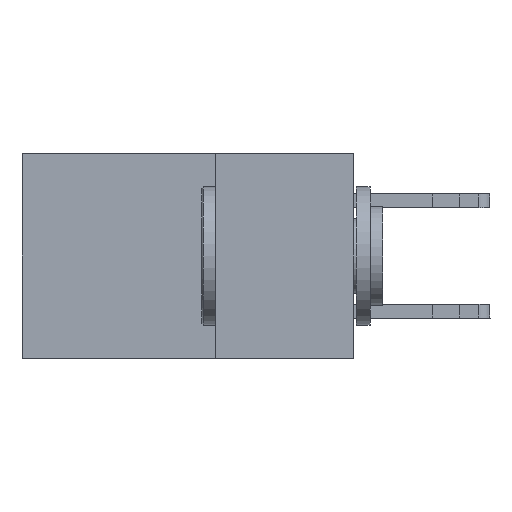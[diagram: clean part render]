
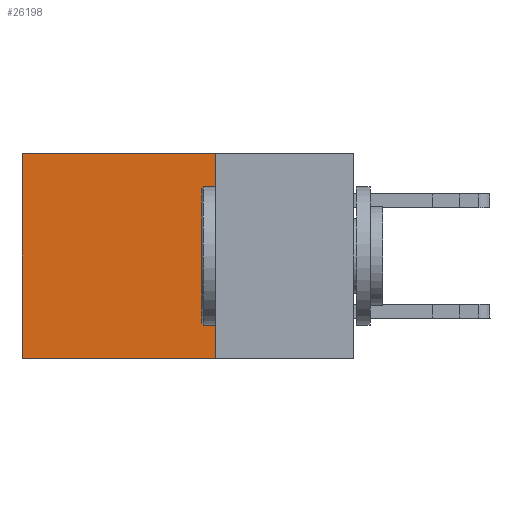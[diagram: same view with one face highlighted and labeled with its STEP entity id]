
A CAD part, left-side view. The second image highlights one B-rep face of the part: STEP entity #26198.
In plain terms, the highlighted planar face has unit normal (-1, 0, 0).
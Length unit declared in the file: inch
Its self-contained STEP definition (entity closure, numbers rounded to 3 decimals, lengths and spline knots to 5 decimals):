
#371 = CARTESIAN_POINT ( 'NONE',  ( 0.2875, 0.25, 0. ) ) ;
#1113 = LINE ( 'NONE', #1233, #7496 ) ;
#1233 = CARTESIAN_POINT ( 'NONE',  ( 0.2875, 0.6, 0. ) ) ;
#1409 = VERTEX_POINT ( 'NONE', #371 ) ;
#1474 = EDGE_CURVE ( 'NONE', #1409, #21731, #23817, .T. ) ;
#1758 = DIRECTION ( 'NONE',  ( 0., 1., 0. ) ) ;
#2656 = VERTEX_POINT ( 'NONE', #4469 ) ;
#2850 = DIRECTION ( 'NONE',  ( 0., 0., -1. ) ) ;
#3101 = LINE ( 'NONE', #16867, #10256 ) ;
#4096 = CARTESIAN_POINT ( 'NONE',  ( 0.2875, 0.25, -0.37 ) ) ;
#4252 = LINE ( 'NONE', #26974, #12473 ) ;
#4469 = CARTESIAN_POINT ( 'NONE',  ( 0.2875, 0.6, -0.37 ) ) ;
#6665 = DIRECTION ( 'NONE',  ( 0., 0., -1. ) ) ;
#7496 = VECTOR ( 'NONE', #10695, 39.37008 ) ;
#10256 = VECTOR ( 'NONE', #14229, 39.37008 ) ;
#10449 = AXIS2_PLACEMENT_3D ( 'NONE', #13661, #18017, #6665 ) ;
#10480 = ORIENTED_EDGE ( 'NONE', *, *, #26735, .F. ) ;
#10695 = DIRECTION ( 'NONE',  ( 0., 0., -1. ) ) ;
#11400 = EDGE_CURVE ( 'NONE', #28031, #2656, #1113, .T. ) ;
#12473 = VECTOR ( 'NONE', #1758, 39.37008 ) ;
#13661 = CARTESIAN_POINT ( 'NONE',  ( 0.2875, 0.25, 0. ) ) ;
#14229 = DIRECTION ( 'NONE',  ( 0., 1., 0. ) ) ;
#16867 = CARTESIAN_POINT ( 'NONE',  ( 0.2875, 0.25, 0. ) ) ;
#17924 = PLANE ( 'NONE',  #10449 ) ;
#18017 = DIRECTION ( 'NONE',  ( 1., 0., 0. ) ) ;
#19285 = EDGE_CURVE ( 'NONE', #1409, #28031, #3101, .T. ) ;
#20119 = ORIENTED_EDGE ( 'NONE', *, *, #1474, .F. ) ;
#21731 = VERTEX_POINT ( 'NONE', #4096 ) ;
#22331 = CARTESIAN_POINT ( 'NONE',  ( 0.2875, 0.6, 0. ) ) ;
#23463 = VECTOR ( 'NONE', #2850, 39.37008 ) ;
#23692 = CARTESIAN_POINT ( 'NONE',  ( 0.2875, 0.25, 0. ) ) ;
#23817 = LINE ( 'NONE', #23692, #23463 ) ;
#26198 = ADVANCED_FACE ( 'NONE', ( #27197 ), #17924, .F. ) ;
#26735 = EDGE_CURVE ( 'NONE', #21731, #2656, #4252, .T. ) ;
#26974 = CARTESIAN_POINT ( 'NONE',  ( 0.2875, 0.25, -0.37 ) ) ;
#27197 = FACE_OUTER_BOUND ( 'NONE', #29505, .T. ) ;
#28031 = VERTEX_POINT ( 'NONE', #22331 ) ;
#28816 = ORIENTED_EDGE ( 'NONE', *, *, #11400, .T. ) ;
#29505 = EDGE_LOOP ( 'NONE', ( #28816, #10480, #20119, #29571 ) ) ;
#29571 = ORIENTED_EDGE ( 'NONE', *, *, #19285, .T. ) ;
